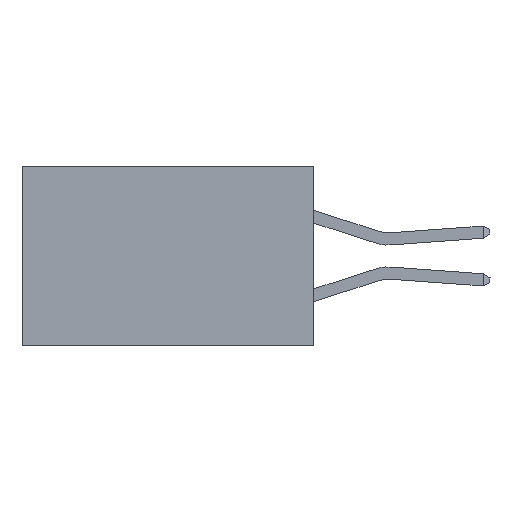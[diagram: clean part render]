
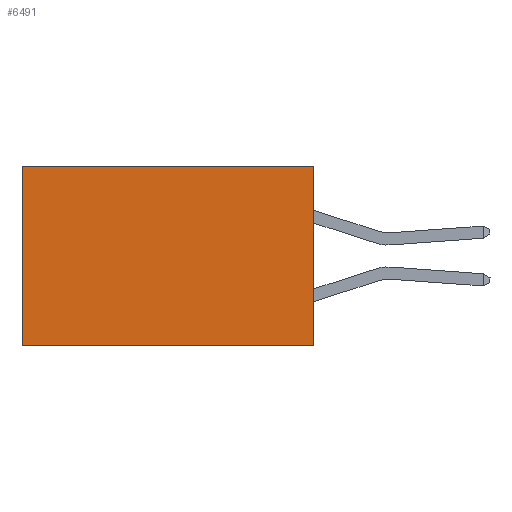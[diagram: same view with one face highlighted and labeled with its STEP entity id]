
A CAD part, left-side view. The second image highlights one B-rep face of the part: STEP entity #6491.
In plain terms, the highlighted planar face has unit normal (-1, 0, 0).
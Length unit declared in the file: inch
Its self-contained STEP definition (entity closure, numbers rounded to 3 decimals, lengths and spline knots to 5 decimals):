
#195 = LINE ( 'NONE', #1140, #27222 ) ;
#286 = EDGE_CURVE ( 'NONE', #426, #6050, #195, .T. ) ;
#409 = DIRECTION ( 'NONE',  ( 0., 1., 0. ) ) ;
#426 = VERTEX_POINT ( 'NONE', #18244 ) ;
#741 = EDGE_CURVE ( 'NONE', #18023, #6050, #23340, .T. ) ;
#1140 = CARTESIAN_POINT ( 'NONE',  ( 0.2875, 0., -0.37 ) ) ;
#3098 = VECTOR ( 'NONE', #409, 39.37008 ) ;
#3598 = CARTESIAN_POINT ( 'NONE',  ( 0.2875, 0.6, -0.37 ) ) ;
#5262 = DIRECTION ( 'NONE',  ( 0., 0., -1. ) ) ;
#6050 = VERTEX_POINT ( 'NONE', #3598 ) ;
#6491 = ADVANCED_FACE ( 'NONE', ( #9327 ), #12209, .F. ) ;
#6642 = EDGE_CURVE ( 'NONE', #21476, #426, #24383, .T. ) ;
#6910 = EDGE_LOOP ( 'NONE', ( #9996, #27377, #27529, #21684 ) ) ;
#9327 = FACE_OUTER_BOUND ( 'NONE', #6910, .T. ) ;
#9459 = CARTESIAN_POINT ( 'NONE',  ( 0.2875, 0.6, 0. ) ) ;
#9996 = ORIENTED_EDGE ( 'NONE', *, *, #741, .T. ) ;
#10762 = LINE ( 'NONE', #25934, #3098 ) ;
#11993 = VECTOR ( 'NONE', #5262, 39.37008 ) ;
#12209 = PLANE ( 'NONE',  #14962 ) ;
#13193 = EDGE_CURVE ( 'NONE', #21476, #18023, #10762, .T. ) ;
#14698 = DIRECTION ( 'NONE',  ( 0., 0., -1. ) ) ;
#14962 = AXIS2_PLACEMENT_3D ( 'NONE', #16496, #26757, #22562 ) ;
#16496 = CARTESIAN_POINT ( 'NONE',  ( 0.2875, 0., 0. ) ) ;
#18023 = VERTEX_POINT ( 'NONE', #19206 ) ;
#18244 = CARTESIAN_POINT ( 'NONE',  ( 0.2875, 0., -0.37 ) ) ;
#19206 = CARTESIAN_POINT ( 'NONE',  ( 0.2875, 0.6, 0. ) ) ;
#21476 = VERTEX_POINT ( 'NONE', #26033 ) ;
#21684 = ORIENTED_EDGE ( 'NONE', *, *, #13193, .T. ) ;
#22562 = DIRECTION ( 'NONE',  ( 0., 0., -1. ) ) ;
#23340 = LINE ( 'NONE', #9459, #11993 ) ;
#24383 = LINE ( 'NONE', #25357, #26700 ) ;
#24594 = DIRECTION ( 'NONE',  ( 0., 1., 0. ) ) ;
#25357 = CARTESIAN_POINT ( 'NONE',  ( 0.2875, 0., 0. ) ) ;
#25934 = CARTESIAN_POINT ( 'NONE',  ( 0.2875, 0., 0. ) ) ;
#26033 = CARTESIAN_POINT ( 'NONE',  ( 0.2875, 0., 0. ) ) ;
#26700 = VECTOR ( 'NONE', #14698, 39.37008 ) ;
#26757 = DIRECTION ( 'NONE',  ( 1., 0., 0. ) ) ;
#27222 = VECTOR ( 'NONE', #24594, 39.37008 ) ;
#27377 = ORIENTED_EDGE ( 'NONE', *, *, #286, .F. ) ;
#27529 = ORIENTED_EDGE ( 'NONE', *, *, #6642, .F. ) ;
